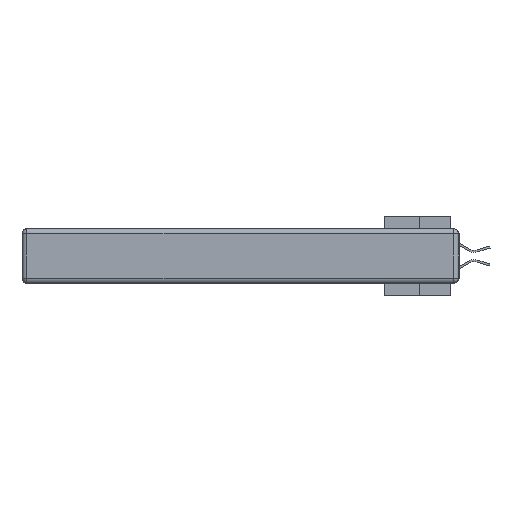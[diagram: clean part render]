
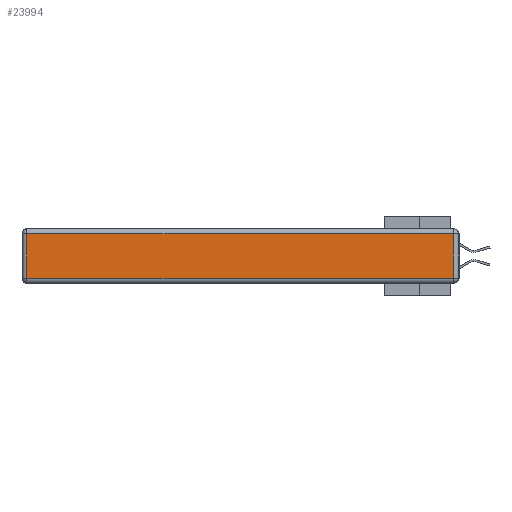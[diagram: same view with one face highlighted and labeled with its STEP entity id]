
A CAD part, left-side view. The second image highlights one B-rep face of the part: STEP entity #23994.
In plain terms, the highlighted planar face has unit normal (-1, 0, 0).
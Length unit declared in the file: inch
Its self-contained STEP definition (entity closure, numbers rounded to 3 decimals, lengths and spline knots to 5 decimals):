
#1398 = VECTOR ( 'NONE', #9732, 39.37008 ) ;
#1406 = VERTEX_POINT ( 'NONE', #24803 ) ;
#1747 = CARTESIAN_POINT ( 'NONE',  ( 0., 0., -0.313 ) ) ;
#1980 = CARTESIAN_POINT ( 'NONE',  ( 0., 2.72, -0.313 ) ) ;
#2557 = CARTESIAN_POINT ( 'NONE',  ( 0., 2.72, -0.03 ) ) ;
#2632 = VERTEX_POINT ( 'NONE', #23354 ) ;
#3633 = VECTOR ( 'NONE', #32186, 39.37008 ) ;
#4135 = DIRECTION ( 'NONE',  ( 0., -1., 0. ) ) ;
#4807 = ORIENTED_EDGE ( 'NONE', *, *, #25837, .T. ) ;
#6731 = LINE ( 'NONE', #26457, #3633 ) ;
#7475 = ORIENTED_EDGE ( 'NONE', *, *, #29675, .T. ) ;
#9584 = PLANE ( 'NONE',  #25475 ) ;
#9732 = DIRECTION ( 'NONE',  ( 0., 0., 1. ) ) ;
#11035 = VECTOR ( 'NONE', #28923, 39.37008 ) ;
#12534 = DIRECTION ( 'NONE',  ( 0., 0., 1. ) ) ;
#14032 = EDGE_CURVE ( 'NONE', #1406, #30881, #6731, .T. ) ;
#14285 = VECTOR ( 'NONE', #4135, 39.37008 ) ;
#17672 = CARTESIAN_POINT ( 'NONE',  ( 0., 2.72, -0.343 ) ) ;
#17902 = ORIENTED_EDGE ( 'NONE', *, *, #14032, .T. ) ;
#19606 = ORIENTED_EDGE ( 'NONE', *, *, #35424, .T. ) ;
#19683 = EDGE_LOOP ( 'NONE', ( #7475, #4807, #17902, #19606 ) ) ;
#21001 = VERTEX_POINT ( 'NONE', #1980 ) ;
#23354 = CARTESIAN_POINT ( 'NONE',  ( 0., 0.03, -0.313 ) ) ;
#23580 = DIRECTION ( 'NONE',  ( -1., 0., 0. ) ) ;
#23994 = ADVANCED_FACE ( 'NONE', ( #29115 ), #9584, .T. ) ;
#24803 = CARTESIAN_POINT ( 'NONE',  ( 0., 0.03, -0.03 ) ) ;
#25475 = AXIS2_PLACEMENT_3D ( 'NONE', #34634, #23580, #12534 ) ;
#25837 = EDGE_CURVE ( 'NONE', #2632, #1406, #31855, .T. ) ;
#26457 = CARTESIAN_POINT ( 'NONE',  ( 0., 2.75, -0.03 ) ) ;
#28923 = DIRECTION ( 'NONE',  ( 0., 0., -1. ) ) ;
#29115 = FACE_OUTER_BOUND ( 'NONE', #19683, .T. ) ;
#29675 = EDGE_CURVE ( 'NONE', #21001, #2632, #32732, .T. ) ;
#30881 = VERTEX_POINT ( 'NONE', #2557 ) ;
#31855 = LINE ( 'NONE', #34958, #1398 ) ;
#32186 = DIRECTION ( 'NONE',  ( 0., 1., 0. ) ) ;
#32732 = LINE ( 'NONE', #1747, #14285 ) ;
#33900 = LINE ( 'NONE', #17672, #11035 ) ;
#34634 = CARTESIAN_POINT ( 'NONE',  ( 0., 0., -0.343 ) ) ;
#34958 = CARTESIAN_POINT ( 'NONE',  ( 0., 0.03, -0.343 ) ) ;
#35424 = EDGE_CURVE ( 'NONE', #30881, #21001, #33900, .T. ) ;
